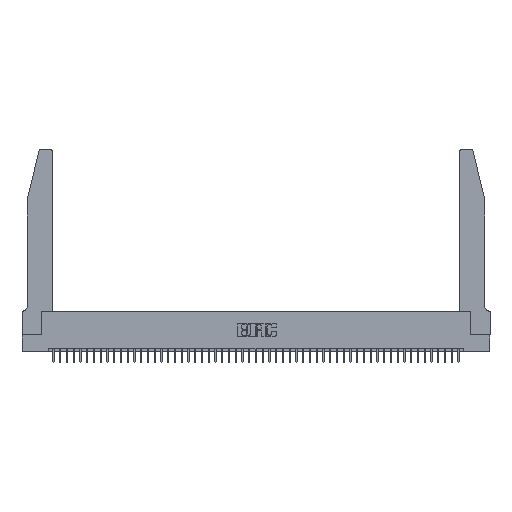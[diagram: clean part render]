
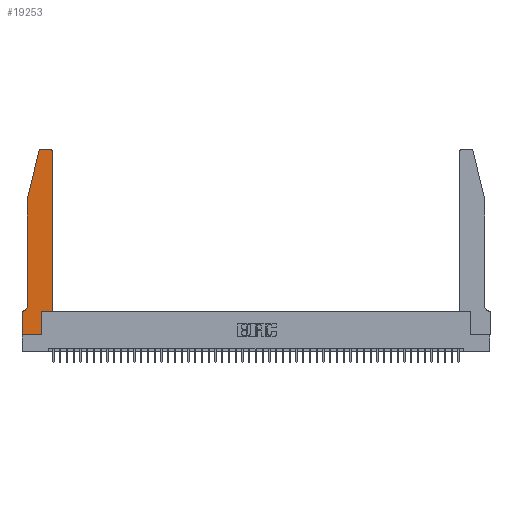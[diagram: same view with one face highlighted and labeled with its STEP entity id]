
A CAD part, top view. The second image highlights one B-rep face of the part: STEP entity #19253.
In plain terms, the highlighted planar face has unit normal (0, 0, 1).
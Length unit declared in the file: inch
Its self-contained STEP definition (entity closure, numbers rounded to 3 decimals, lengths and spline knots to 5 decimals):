
#682 = PLANE ( 'NONE',  #34936 ) ;
#1013 = CARTESIAN_POINT ( 'NONE',  ( 0.284, 2.75, 0.37 ) ) ;
#2782 = DIRECTION ( 'NONE',  ( 1., 0., 0. ) ) ;
#3536 = ORIENTED_EDGE ( 'NONE', *, *, #28280, .T. ) ;
#4795 = CARTESIAN_POINT ( 'NONE',  ( 0., 0., 0.37 ) ) ;
#4982 = EDGE_LOOP ( 'NONE', ( #18640, #49649, #33684, #12659, #9777, #45195, #8517, #3536, #17135, #11170, #42381, #45568 ) ) ;
#5358 = DIRECTION ( 'NONE',  ( 0., 1., 0. ) ) ;
#5820 = EDGE_CURVE ( 'NONE', #23497, #21525, #19964, .T. ) ;
#6084 = VECTOR ( 'NONE', #46510, 39.37008 ) ;
#6606 = VECTOR ( 'NONE', #15110, 39.37008 ) ;
#7127 = DIRECTION ( 'NONE',  ( 1., 0., 0. ) ) ;
#8517 = ORIENTED_EDGE ( 'NONE', *, *, #45423, .T. ) ;
#8538 = EDGE_CURVE ( 'NONE', #24022, #23497, #11888, .T. ) ;
#8822 = VERTEX_POINT ( 'NONE', #44997 ) ;
#9326 = VERTEX_POINT ( 'NONE', #41825 ) ;
#9777 = ORIENTED_EDGE ( 'NONE', *, *, #8538, .T. ) ;
#10924 = CARTESIAN_POINT ( 'NONE',  ( 0.4505, 0.35, 0.37 ) ) ;
#11170 = ORIENTED_EDGE ( 'NONE', *, *, #16800, .T. ) ;
#11399 = CARTESIAN_POINT ( 'NONE',  ( 0., 0., 0.37 ) ) ;
#11663 = DIRECTION ( 'NONE',  ( 1., 0., 0. ) ) ;
#11888 = CIRCLE ( 'NONE', #12988, 0.07 ) ;
#12369 = CARTESIAN_POINT ( 'NONE',  ( 0., 0.35, 0.37 ) ) ;
#12659 = ORIENTED_EDGE ( 'NONE', *, *, #24088, .T. ) ;
#12988 = AXIS2_PLACEMENT_3D ( 'NONE', #16105, #47111, #24035 ) ;
#14712 = FACE_OUTER_BOUND ( 'NONE', #4982, .T. ) ;
#15110 = DIRECTION ( 'NONE',  ( 0., -1., 0. ) ) ;
#16105 = CARTESIAN_POINT ( 'NONE',  ( 0.0055, 0.42, 0.37 ) ) ;
#16177 = VERTEX_POINT ( 'NONE', #44844 ) ;
#16800 = EDGE_CURVE ( 'NONE', #19477, #45580, #26365, .T. ) ;
#17135 = ORIENTED_EDGE ( 'NONE', *, *, #38840, .T. ) ;
#18457 = DIRECTION ( 'NONE',  ( 0., -1., 0. ) ) ;
#18640 = ORIENTED_EDGE ( 'NONE', *, *, #27028, .T. ) ;
#19253 = ADVANCED_FACE ( 'NONE', ( #14712 ), #682, .T. ) ;
#19325 = CARTESIAN_POINT ( 'NONE',  ( 0.4505, 0.35, 0.37 ) ) ;
#19477 = VERTEX_POINT ( 'NONE', #44351 ) ;
#19964 = LINE ( 'NONE', #38006, #47883 ) ;
#20007 = CARTESIAN_POINT ( 'NONE',  ( 0.4505, 2.72, 0.37 ) ) ;
#20877 = CARTESIAN_POINT ( 'NONE',  ( 0.25487, 2.72718, 0.37 ) ) ;
#21087 = VECTOR ( 'NONE', #5358, 39.37008 ) ;
#21525 = VERTEX_POINT ( 'NONE', #28511 ) ;
#21756 = EDGE_CURVE ( 'NONE', #45580, #49715, #48394, .T. ) ;
#23102 = EDGE_CURVE ( 'NONE', #49715, #9326, #35252, .T. ) ;
#23357 = CARTESIAN_POINT ( 'NONE',  ( 0.284, 2.72, 0.37 ) ) ;
#23497 = VERTEX_POINT ( 'NONE', #37155 ) ;
#24022 = VERTEX_POINT ( 'NONE', #24888 ) ;
#24035 = DIRECTION ( 'NONE',  ( -1., 0., 0. ) ) ;
#24088 = EDGE_CURVE ( 'NONE', #8822, #24022, #43075, .T. ) ;
#24553 = CARTESIAN_POINT ( 'NONE',  ( 0.0755, 2., 0.37 ) ) ;
#24888 = CARTESIAN_POINT ( 'NONE',  ( 0.0755, 0.42, 0.37 ) ) ;
#25919 = EDGE_CURVE ( 'NONE', #41872, #39521, #32500, .T. ) ;
#26063 = LINE ( 'NONE', #46349, #6084 ) ;
#26365 = LINE ( 'NONE', #10924, #48244 ) ;
#27028 = EDGE_CURVE ( 'NONE', #9326, #41872, #45861, .T. ) ;
#27748 = VECTOR ( 'NONE', #45463, 39.37008 ) ;
#28280 = EDGE_CURVE ( 'NONE', #45573, #16177, #49953, .T. ) ;
#28361 = CARTESIAN_POINT ( 'NONE',  ( 0.2865, 0.35, 0.37 ) ) ;
#28511 = CARTESIAN_POINT ( 'NONE',  ( 0., 0.35, 0.37 ) ) ;
#29450 = EDGE_CURVE ( 'NONE', #39521, #8822, #26063, .T. ) ;
#29506 = LINE ( 'NONE', #28361, #21087 ) ;
#29955 = DIRECTION ( 'NONE',  ( 0., 0., 1. ) ) ;
#30072 = VECTOR ( 'NONE', #43150, 39.37008 ) ;
#30810 = DIRECTION ( 'NONE',  ( 1., 0., 0. ) ) ;
#30887 = CARTESIAN_POINT ( 'NONE',  ( 0.4205, 2.72, 0.37 ) ) ;
#32500 = CIRCLE ( 'NONE', #38070, 0.03 ) ;
#33684 = ORIENTED_EDGE ( 'NONE', *, *, #29450, .T. ) ;
#34418 = CARTESIAN_POINT ( 'NONE',  ( 0.4505, 0.35, 0.37 ) ) ;
#34936 = AXIS2_PLACEMENT_3D ( 'NONE', #12369, #43334, #39802 ) ;
#35252 = CIRCLE ( 'NONE', #39679, 0.03 ) ;
#35416 = VECTOR ( 'NONE', #7127, 39.37008 ) ;
#35814 = VECTOR ( 'NONE', #18457, 39.37008 ) ;
#37155 = CARTESIAN_POINT ( 'NONE',  ( 0.0055, 0.35, 0.37 ) ) ;
#38006 = CARTESIAN_POINT ( 'NONE',  ( 0.0755, 0.35, 0.37 ) ) ;
#38070 = AXIS2_PLACEMENT_3D ( 'NONE', #23357, #29955, #30810 ) ;
#38840 = EDGE_CURVE ( 'NONE', #16177, #19477, #29506, .T. ) ;
#39521 = VERTEX_POINT ( 'NONE', #20877 ) ;
#39679 = AXIS2_PLACEMENT_3D ( 'NONE', #30887, #42120, #11663 ) ;
#39802 = DIRECTION ( 'NONE',  ( 1., 0., 0. ) ) ;
#41421 = DIRECTION ( 'NONE',  ( -1., 0., 0. ) ) ;
#41825 = CARTESIAN_POINT ( 'NONE',  ( 0.4205, 2.75, 0.37 ) ) ;
#41872 = VERTEX_POINT ( 'NONE', #1013 ) ;
#42120 = DIRECTION ( 'NONE',  ( 0., 0., 1. ) ) ;
#42381 = ORIENTED_EDGE ( 'NONE', *, *, #21756, .T. ) ;
#43075 = LINE ( 'NONE', #24553, #35814 ) ;
#43150 = DIRECTION ( 'NONE',  ( -1., 0., 0. ) ) ;
#43334 = DIRECTION ( 'NONE',  ( 0., 0., 1. ) ) ;
#43496 = CARTESIAN_POINT ( 'NONE',  ( 0.2605, 2.75, 0.37 ) ) ;
#44351 = CARTESIAN_POINT ( 'NONE',  ( 0.2865, 0.35, 0.37 ) ) ;
#44844 = CARTESIAN_POINT ( 'NONE',  ( 0.2865, 0., 0.37 ) ) ;
#44997 = CARTESIAN_POINT ( 'NONE',  ( 0.0755, 2., 0.37 ) ) ;
#45195 = ORIENTED_EDGE ( 'NONE', *, *, #5820, .T. ) ;
#45423 = EDGE_CURVE ( 'NONE', #21525, #45573, #48420, .T. ) ;
#45463 = DIRECTION ( 'NONE',  ( 0., 1., 0. ) ) ;
#45568 = ORIENTED_EDGE ( 'NONE', *, *, #23102, .T. ) ;
#45573 = VERTEX_POINT ( 'NONE', #4795 ) ;
#45580 = VERTEX_POINT ( 'NONE', #19325 ) ;
#45861 = LINE ( 'NONE', #43496, #30072 ) ;
#45943 = CARTESIAN_POINT ( 'NONE',  ( 0., 0., 0.37 ) ) ;
#46349 = CARTESIAN_POINT ( 'NONE',  ( 0.0755, 2., 0.37 ) ) ;
#46510 = DIRECTION ( 'NONE',  ( -0.239, -0.971, 0. ) ) ;
#47111 = DIRECTION ( 'NONE',  ( 0., 0., -1. ) ) ;
#47883 = VECTOR ( 'NONE', #41421, 39.37008 ) ;
#48244 = VECTOR ( 'NONE', #2782, 39.37008 ) ;
#48394 = LINE ( 'NONE', #34418, #27748 ) ;
#48420 = LINE ( 'NONE', #45943, #6606 ) ;
#49649 = ORIENTED_EDGE ( 'NONE', *, *, #25919, .T. ) ;
#49715 = VERTEX_POINT ( 'NONE', #20007 ) ;
#49953 = LINE ( 'NONE', #11399, #35416 ) ;
